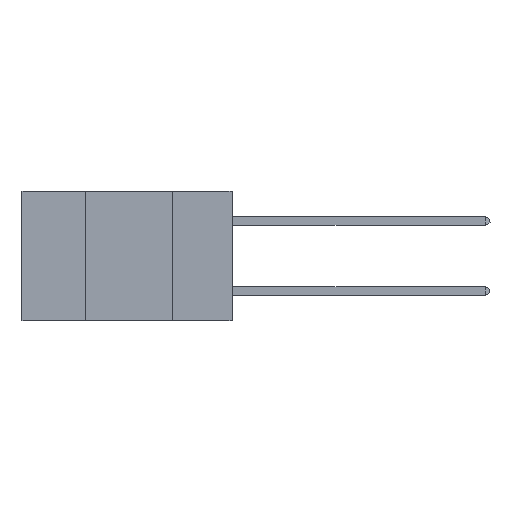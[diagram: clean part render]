
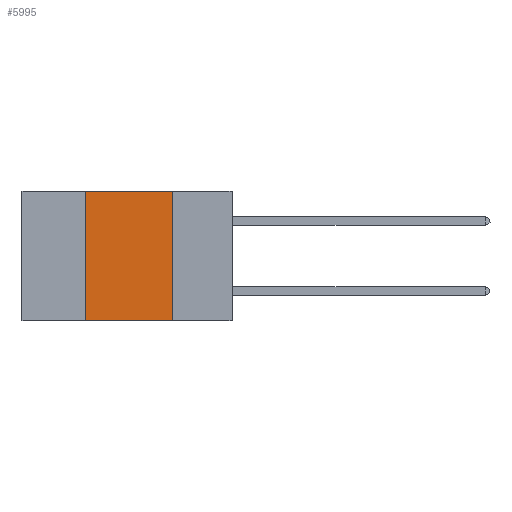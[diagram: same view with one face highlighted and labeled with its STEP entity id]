
A CAD part, left-side view. The second image highlights one B-rep face of the part: STEP entity #5995.
In plain terms, the highlighted planar face has unit normal (-1, 0, 0).
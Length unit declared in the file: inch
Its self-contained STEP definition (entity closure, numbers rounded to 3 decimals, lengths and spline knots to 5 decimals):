
#12 = LINE ( 'NONE', #19736, #11773 ) ;
#172 = VECTOR ( 'NONE', #3869, 39.37008 ) ;
#506 = CARTESIAN_POINT ( 'NONE',  ( 0., 0.42, 0. ) ) ;
#1585 = EDGE_CURVE ( 'NONE', #23786, #15177, #16085, .T. ) ;
#2188 = ORIENTED_EDGE ( 'NONE', *, *, #1585, .F. ) ;
#2215 = DIRECTION ( 'NONE',  ( 0., -1., 0. ) ) ;
#2581 = DIRECTION ( 'NONE',  ( 0., -1., 0. ) ) ;
#3869 = DIRECTION ( 'NONE',  ( 0., 0., 1. ) ) ;
#4350 = ORIENTED_EDGE ( 'NONE', *, *, #24096, .F. ) ;
#4384 = CARTESIAN_POINT ( 'NONE',  ( 0., 0.6, 0. ) ) ;
#5247 = VERTEX_POINT ( 'NONE', #10192 ) ;
#5355 = CARTESIAN_POINT ( 'NONE',  ( 0., 0.17, 0. ) ) ;
#5819 = LINE ( 'NONE', #5355, #9061 ) ;
#5995 = ADVANCED_FACE ( 'NONE', ( #9093 ), #14511, .F. ) ;
#9061 = VECTOR ( 'NONE', #18526, 39.37008 ) ;
#9093 = FACE_OUTER_BOUND ( 'NONE', #16061, .T. ) ;
#9852 = ORIENTED_EDGE ( 'NONE', *, *, #15235, .F. ) ;
#10192 = CARTESIAN_POINT ( 'NONE',  ( 0., 0.17, 0. ) ) ;
#10672 = DIRECTION ( 'NONE',  ( 0., 0., -1. ) ) ;
#11077 = LINE ( 'NONE', #4384, #21988 ) ;
#11773 = VECTOR ( 'NONE', #2581, 39.37008 ) ;
#12039 = CARTESIAN_POINT ( 'NONE',  ( 0., 0.17, -0.37 ) ) ;
#13481 = CARTESIAN_POINT ( 'NONE',  ( 0., 0.42, 0. ) ) ;
#14511 = PLANE ( 'NONE',  #14661 ) ;
#14661 = AXIS2_PLACEMENT_3D ( 'NONE', #14845, #18596, #10672 ) ;
#14845 = CARTESIAN_POINT ( 'NONE',  ( 0., 0.6, 0. ) ) ;
#15177 = VERTEX_POINT ( 'NONE', #506 ) ;
#15235 = EDGE_CURVE ( 'NONE', #15177, #5247, #11077, .T. ) ;
#16061 = EDGE_LOOP ( 'NONE', ( #4350, #9852, #2188, #16614 ) ) ;
#16085 = LINE ( 'NONE', #13481, #172 ) ;
#16614 = ORIENTED_EDGE ( 'NONE', *, *, #23102, .T. ) ;
#16956 = VERTEX_POINT ( 'NONE', #12039 ) ;
#18526 = DIRECTION ( 'NONE',  ( 0., 0., -1. ) ) ;
#18596 = DIRECTION ( 'NONE',  ( 1., 0., 0. ) ) ;
#19116 = CARTESIAN_POINT ( 'NONE',  ( 0., 0.42, -0.37 ) ) ;
#19736 = CARTESIAN_POINT ( 'NONE',  ( 0., 0.6, -0.37 ) ) ;
#21988 = VECTOR ( 'NONE', #2215, 39.37008 ) ;
#23102 = EDGE_CURVE ( 'NONE', #23786, #16956, #12, .T. ) ;
#23786 = VERTEX_POINT ( 'NONE', #19116 ) ;
#24096 = EDGE_CURVE ( 'NONE', #5247, #16956, #5819, .T. ) ;
